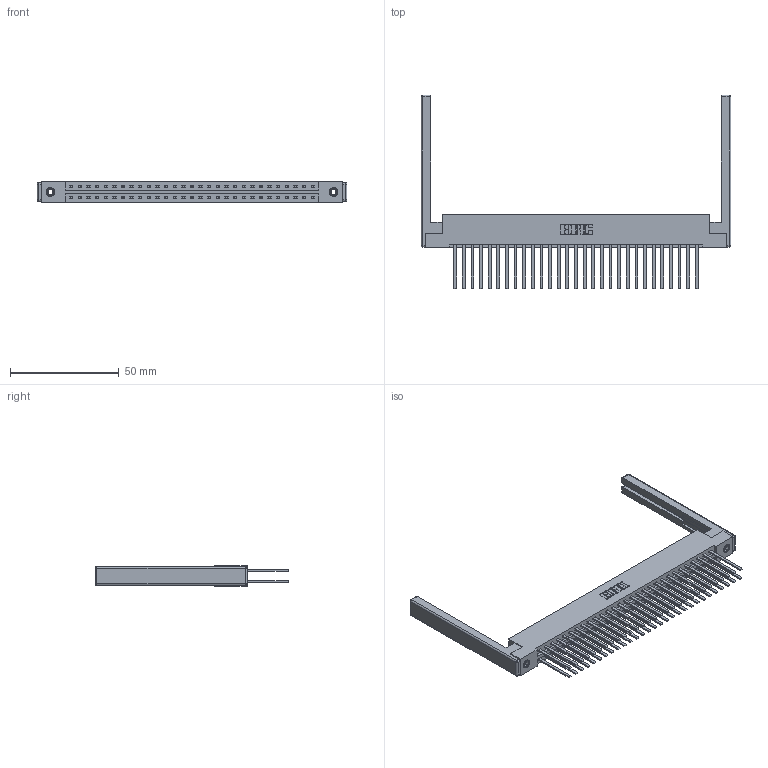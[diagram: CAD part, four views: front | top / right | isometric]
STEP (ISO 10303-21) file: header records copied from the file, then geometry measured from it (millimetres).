
FILE_DESCRIPTION (( 'STEP AP203' ), '1' );
FILE_NAME ('337-058-544-268.STEP', '2019-10-09T19:52:39', ( '' ), ( '' ), 'SwSTEP 2.0', 'SolidWorks 2016', '' );
FILE_SCHEMA (( 'CONFIG_CONTROL_DESIGN' ));
Length unit declared in the file: inch
Products named in the file (5): 307-220-068; 337 Part_Flush Mounting Lugs - 0.156 Dia-TI; 345-250-001_345-250-001-102; 345-292-001_345-293-144; 337-058-544-268
Assembly tree (63 placements, depth 2):
  337-058-544-268
    337 Part_Flush Mounting Lugs - 0.156 Dia-TI
    345-292-001_345-293-144  x58
    345-250-001_345-250-001-102  x2
    307-220-068  x2
Bounding box: 142.34 x 89.03 x 9.4 mm (x, y, z)
Volume: 20025.9 mm3; surface area: 24246.4 mm2
Topology: 63 solids, 63 shells, 3052 faces, 8995 edges, 5898 vertices
Faces by surface type: plane 2130, cylinder 898, cone 12, sphere 8, torus 4
Entity records: 26742 total; most frequent: CARTESIAN_POINT 4479, ORIENTED_EDGE 4404, DIRECTION 3900, EDGE_CURVE 2202, VECTOR 2028, LINE 2028, VERTEX_POINT 1458, AXIS2_PLACEMENT_3D 936
